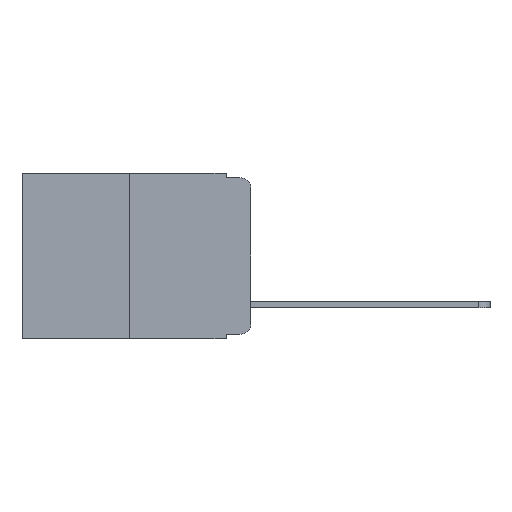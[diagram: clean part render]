
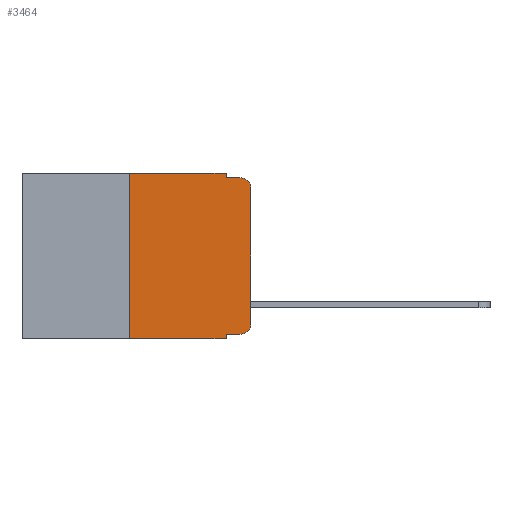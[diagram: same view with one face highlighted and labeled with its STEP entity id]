
A CAD part, left-side view. The second image highlights one B-rep face of the part: STEP entity #3464.
In plain terms, the highlighted planar face has unit normal (-1, 0, 0).
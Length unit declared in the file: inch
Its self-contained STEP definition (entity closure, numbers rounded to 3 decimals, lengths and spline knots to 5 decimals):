
#1002 = FACE_OUTER_BOUND ( 'NONE', #7676, .T. ) ;
#1256 = VERTEX_POINT ( 'NONE', #10761 ) ;
#1452 = VERTEX_POINT ( 'NONE', #2052 ) ;
#1521 = VECTOR ( 'NONE', #17014, 39.37008 ) ;
#2052 = CARTESIAN_POINT ( 'NONE',  ( 0., 0.051, 0. ) ) ;
#2286 = EDGE_CURVE ( 'NONE', #4171, #13737, #6311, .T. ) ;
#2509 = VECTOR ( 'NONE', #10797, 39.37008 ) ;
#2576 = EDGE_CURVE ( 'NONE', #1452, #9476, #3463, .T. ) ;
#2688 = ORIENTED_EDGE ( 'NONE', *, *, #2286, .F. ) ;
#2738 = DIRECTION ( 'NONE',  ( -1., 0., 0. ) ) ;
#2751 = CARTESIAN_POINT ( 'NONE',  ( 0., 0.02, -0.333 ) ) ;
#3301 = LINE ( 'NONE', #17503, #6385 ) ;
#3403 = CIRCLE ( 'NONE', #14250, 0.02 ) ;
#3463 = LINE ( 'NONE', #13765, #1521 ) ;
#3464 = ADVANCED_FACE ( 'NONE', ( #1002 ), #17925, .F. ) ;
#3527 = LINE ( 'NONE', #15789, #18822 ) ;
#3554 = CARTESIAN_POINT ( 'NONE',  ( 0., 0.473, -0.343 ) ) ;
#3816 = EDGE_CURVE ( 'NONE', #9476, #14162, #16804, .T. ) ;
#4171 = VERTEX_POINT ( 'NONE', #11186 ) ;
#4298 = ORIENTED_EDGE ( 'NONE', *, *, #19790, .T. ) ;
#4491 = ORIENTED_EDGE ( 'NONE', *, *, #6511, .F. ) ;
#4655 = VERTEX_POINT ( 'NONE', #5470 ) ;
#4997 = VERTEX_POINT ( 'NONE', #11705 ) ;
#5324 = DIRECTION ( 'NONE',  ( 0., -1., 0. ) ) ;
#5446 = VECTOR ( 'NONE', #8072, 39.37008 ) ;
#5470 = CARTESIAN_POINT ( 'NONE',  ( 0., 0.051, -0.343 ) ) ;
#5488 = AXIS2_PLACEMENT_3D ( 'NONE', #18057, #14727, #13451 ) ;
#5556 = EDGE_CURVE ( 'NONE', #4997, #14162, #6639, .T. ) ;
#5747 = EDGE_CURVE ( 'NONE', #12866, #17771, #3301, .T. ) ;
#6104 = CARTESIAN_POINT ( 'NONE',  ( 0., 0.051, -0.01 ) ) ;
#6311 = LINE ( 'NONE', #17192, #9689 ) ;
#6385 = VECTOR ( 'NONE', #5324, 39.37008 ) ;
#6441 = CARTESIAN_POINT ( 'NONE',  ( 0., 0.473, 0. ) ) ;
#6511 = EDGE_CURVE ( 'NONE', #13737, #1452, #15755, .T. ) ;
#6639 = CIRCLE ( 'NONE', #19354, 0.02 ) ;
#6721 = DIRECTION ( 'NONE',  ( 0., 0., -1. ) ) ;
#6849 = EDGE_CURVE ( 'NONE', #12866, #4655, #3527, .T. ) ;
#7067 = ORIENTED_EDGE ( 'NONE', *, *, #2576, .F. ) ;
#7116 = DIRECTION ( 'NONE',  ( 0., 0., -1. ) ) ;
#7366 = ORIENTED_EDGE ( 'NONE', *, *, #5747, .T. ) ;
#7676 = EDGE_LOOP ( 'NONE', ( #4298, #8885, #9859, #7067, #4491, #2688, #9888, #12673, #7366, #10996 ) ) ;
#7699 = EDGE_CURVE ( 'NONE', #17771, #1256, #3403, .T. ) ;
#7791 = CARTESIAN_POINT ( 'NONE',  ( 0., 0., 0. ) ) ;
#8072 = DIRECTION ( 'NONE',  ( 0., -1., 0. ) ) ;
#8885 = ORIENTED_EDGE ( 'NONE', *, *, #5556, .T. ) ;
#9476 = VERTEX_POINT ( 'NONE', #6104 ) ;
#9614 = VECTOR ( 'NONE', #17172, 39.37008 ) ;
#9689 = VECTOR ( 'NONE', #11264, 39.37008 ) ;
#9859 = ORIENTED_EDGE ( 'NONE', *, *, #3816, .F. ) ;
#9888 = ORIENTED_EDGE ( 'NONE', *, *, #12161, .T. ) ;
#10761 = CARTESIAN_POINT ( 'NONE',  ( 0., 0., -0.313 ) ) ;
#10797 = DIRECTION ( 'NONE',  ( 0., 0., 1. ) ) ;
#10996 = ORIENTED_EDGE ( 'NONE', *, *, #7699, .T. ) ;
#11186 = CARTESIAN_POINT ( 'NONE',  ( 0., 0.25, -0.343 ) ) ;
#11264 = DIRECTION ( 'NONE',  ( 0., 0., 1. ) ) ;
#11705 = CARTESIAN_POINT ( 'NONE',  ( 0., 0., -0.03 ) ) ;
#12161 = EDGE_CURVE ( 'NONE', #4171, #4655, #17431, .T. ) ;
#12459 = CARTESIAN_POINT ( 'NONE',  ( 0., 0.051, -0.01 ) ) ;
#12673 = ORIENTED_EDGE ( 'NONE', *, *, #6849, .F. ) ;
#12866 = VERTEX_POINT ( 'NONE', #13361 ) ;
#13361 = CARTESIAN_POINT ( 'NONE',  ( 0., 0.051, -0.333 ) ) ;
#13451 = DIRECTION ( 'NONE',  ( 0., 0., -1. ) ) ;
#13649 = DIRECTION ( 'NONE',  ( 0., -1., 0. ) ) ;
#13737 = VERTEX_POINT ( 'NONE', #16669 ) ;
#13765 = CARTESIAN_POINT ( 'NONE',  ( 0., 0.051, 0. ) ) ;
#13998 = LINE ( 'NONE', #7791, #2509 ) ;
#14162 = VERTEX_POINT ( 'NONE', #14852 ) ;
#14250 = AXIS2_PLACEMENT_3D ( 'NONE', #16577, #2738, #14984 ) ;
#14727 = DIRECTION ( 'NONE',  ( 1., 0., 0. ) ) ;
#14852 = CARTESIAN_POINT ( 'NONE',  ( 0., 0.02, -0.01 ) ) ;
#14984 = DIRECTION ( 'NONE',  ( 0., 0., -1. ) ) ;
#15755 = LINE ( 'NONE', #6441, #18818 ) ;
#15789 = CARTESIAN_POINT ( 'NONE',  ( 0., 0.051, 0. ) ) ;
#16493 = CARTESIAN_POINT ( 'NONE',  ( 0., 0.02, -0.03 ) ) ;
#16577 = CARTESIAN_POINT ( 'NONE',  ( 0., 0.02, -0.313 ) ) ;
#16669 = CARTESIAN_POINT ( 'NONE',  ( 0., 0.25, 0. ) ) ;
#16804 = LINE ( 'NONE', #12459, #9614 ) ;
#17014 = DIRECTION ( 'NONE',  ( 0., 0., -1. ) ) ;
#17172 = DIRECTION ( 'NONE',  ( 0., -1., 0. ) ) ;
#17192 = CARTESIAN_POINT ( 'NONE',  ( 0., 0.25, 0. ) ) ;
#17431 = LINE ( 'NONE', #3554, #5446 ) ;
#17503 = CARTESIAN_POINT ( 'NONE',  ( 0., 0.051, -0.333 ) ) ;
#17771 = VERTEX_POINT ( 'NONE', #2751 ) ;
#17925 = PLANE ( 'NONE',  #5488 ) ;
#17964 = DIRECTION ( 'NONE',  ( -1., 0., 0. ) ) ;
#18057 = CARTESIAN_POINT ( 'NONE',  ( 0., 0.473, 0. ) ) ;
#18818 = VECTOR ( 'NONE', #13649, 39.37008 ) ;
#18822 = VECTOR ( 'NONE', #6721, 39.37008 ) ;
#19354 = AXIS2_PLACEMENT_3D ( 'NONE', #16493, #17964, #7116 ) ;
#19790 = EDGE_CURVE ( 'NONE', #1256, #4997, #13998, .T. ) ;
